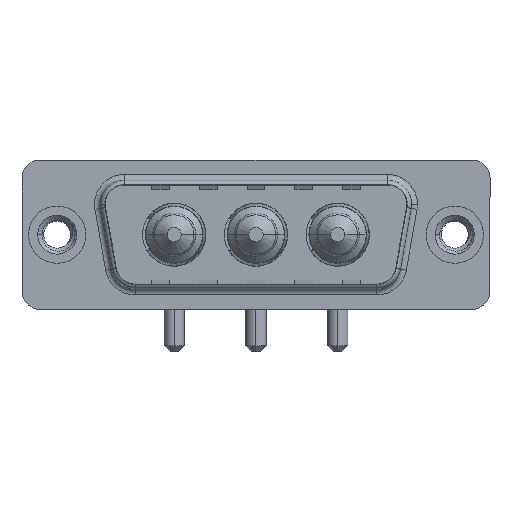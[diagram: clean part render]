
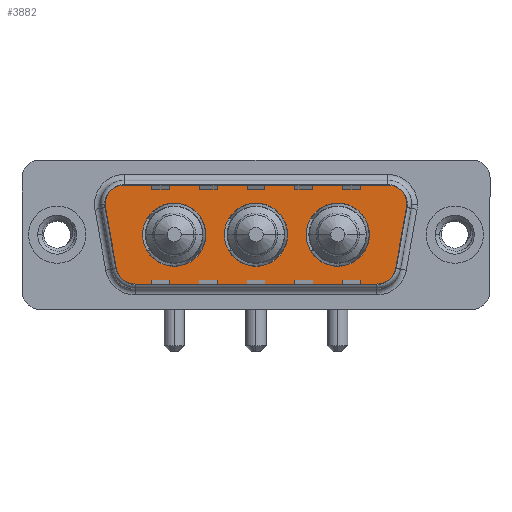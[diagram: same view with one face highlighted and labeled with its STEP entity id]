
A CAD part, top view. The second image highlights one B-rep face of the part: STEP entity #3882.
In plain terms, the highlighted planar face has unit normal (0, 0, 1).
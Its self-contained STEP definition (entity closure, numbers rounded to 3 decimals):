
#53 = VERTEX_POINT ( 'NONE', #10228 ) ;
#57 = CIRCLE ( 'NONE', #4257, 2. ) ;
#200 = LINE ( 'NONE', #8447, #5115 ) ;
#391 = DIRECTION ( 'NONE',  ( 0., 0., 1. ) ) ;
#423 = VERTEX_POINT ( 'NONE', #9043 ) ;
#470 = DIRECTION ( 'NONE',  ( 0., 0., 1. ) ) ;
#472 = ORIENTED_EDGE ( 'NONE', *, *, #7137, .T. ) ;
#653 = DIRECTION ( 'NONE',  ( 1., 0., 0. ) ) ;
#720 = DIRECTION ( 'NONE',  ( 0., 0., 1. ) ) ;
#724 = CARTESIAN_POINT ( 'NONE',  ( 29.889, 2.9, 0. ) ) ;
#821 = DIRECTION ( 'NONE',  ( 0.174, -0.985, 0. ) ) ;
#899 = EDGE_CURVE ( 'NONE', #12222, #423, #8893, .T. ) ;
#1100 = ORIENTED_EDGE ( 'NONE', *, *, #10562, .T. ) ;
#1119 = DIRECTION ( 'NONE',  ( 0., 0., 1. ) ) ;
#1127 = EDGE_CURVE ( 'NONE', #53, #10323, #12072, .T. ) ;
#1172 = VERTEX_POINT ( 'NONE', #9484 ) ;
#1194 = VERTEX_POINT ( 'NONE', #7641 ) ;
#1213 = CARTESIAN_POINT ( 'NONE',  ( 19.3, 0., 0. ) ) ;
#1231 = CARTESIAN_POINT ( 'NONE',  ( 27.889, 2.9, 0. ) ) ;
#1315 = AXIS2_PLACEMENT_3D ( 'NONE', #7459, #3462, #12271 ) ;
#1325 = ORIENTED_EDGE ( 'NONE', *, *, #9516, .T. ) ;
#1352 = DIRECTION ( 'NONE',  ( 0., 0., 1. ) ) ;
#1483 = DIRECTION ( 'NONE',  ( 0., 0., 1. ) ) ;
#1985 = EDGE_LOOP ( 'NONE', ( #4484, #9742, #11621, #472, #1325, #1100, #3845, #10124, #11089 ) ) ;
#2003 = EDGE_CURVE ( 'NONE', #4268, #53, #12152, .T. ) ;
#2082 = EDGE_LOOP ( 'NONE', ( #2613, #12776 ) ) ;
#2243 = CIRCLE ( 'NONE', #12680, 2. ) ;
#2296 = DIRECTION ( 'NONE',  ( 1., 0., 0. ) ) ;
#2495 = EDGE_CURVE ( 'NONE', #10323, #10774, #57, .T. ) ;
#2613 = ORIENTED_EDGE ( 'NONE', *, *, #11477, .F. ) ;
#2951 = CARTESIAN_POINT ( 'NONE',  ( 6.434, -2.9, 0. ) ) ;
#3072 = EDGE_LOOP ( 'NONE', ( #3580, #4823 ) ) ;
#3118 = CARTESIAN_POINT ( 'NONE',  ( 29.859, 2.553, 0. ) ) ;
#3119 = CARTESIAN_POINT ( 'NONE',  ( 27.889, 2.9, 0. ) ) ;
#3271 = VERTEX_POINT ( 'NONE', #10683 ) ;
#3322 = EDGE_CURVE ( 'NONE', #10455, #1172, #9067, .T. ) ;
#3462 = DIRECTION ( 'NONE',  ( 0., 0., 1. ) ) ;
#3522 = VERTEX_POINT ( 'NONE', #5904 ) ;
#3580 = ORIENTED_EDGE ( 'NONE', *, *, #3322, .F. ) ;
#3589 = AXIS2_PLACEMENT_3D ( 'NONE', #9279, #6401, #6276 ) ;
#3667 = CARTESIAN_POINT ( 'NONE',  ( 12.45, 0., 0. ) ) ;
#3845 = ORIENTED_EDGE ( 'NONE', *, *, #899, .T. ) ;
#3882 = ADVANCED_FACE ( 'NONE', ( #8510, #4590, #5574, #10601 ), #12532, .T. ) ;
#4057 = CIRCLE ( 'NONE', #1315, 2.65 ) ;
#4197 = DIRECTION ( 'NONE',  ( -1., 0., 0. ) ) ;
#4220 = DIRECTION ( 'NONE',  ( 0., 0., 1. ) ) ;
#4257 = AXIS2_PLACEMENT_3D ( 'NONE', #3119, #1352, #7123 ) ;
#4268 = VERTEX_POINT ( 'NONE', #12233 ) ;
#4284 = CARTESIAN_POINT ( 'NONE',  ( 26.866, -2.9, 0. ) ) ;
#4433 = VECTOR ( 'NONE', #821, 1000. ) ;
#4484 = ORIENTED_EDGE ( 'NONE', *, *, #2003, .T. ) ;
#4590 = FACE_BOUND ( 'NONE', #2082, .T. ) ;
#4734 = CARTESIAN_POINT ( 'NONE',  ( 23.5, 0., 0. ) ) ;
#4823 = ORIENTED_EDGE ( 'NONE', *, *, #5151, .F. ) ;
#4904 = AXIS2_PLACEMENT_3D ( 'NONE', #4734, #720, #5718 ) ;
#4974 = CARTESIAN_POINT ( 'NONE',  ( 3.441, 2.553, 0. ) ) ;
#5115 = VECTOR ( 'NONE', #6367, 1000. ) ;
#5151 = EDGE_CURVE ( 'NONE', #1172, #10455, #9544, .T. ) ;
#5320 = VERTEX_POINT ( 'NONE', #3667 ) ;
#5481 = AXIS2_PLACEMENT_3D ( 'NONE', #2951, #10925, #9769 ) ;
#5530 = CARTESIAN_POINT ( 'NONE',  ( 7.15, 0., 0. ) ) ;
#5574 = FACE_BOUND ( 'NONE', #6888, .T. ) ;
#5718 = DIRECTION ( 'NONE',  ( 1., 0., 0. ) ) ;
#5741 = VERTEX_POINT ( 'NONE', #7328 ) ;
#5904 = CARTESIAN_POINT ( 'NONE',  ( 27.889, 4.9, 0. ) ) ;
#5947 = AXIS2_PLACEMENT_3D ( 'NONE', #7454, #10639, #11424 ) ;
#6118 = CARTESIAN_POINT ( 'NONE',  ( 16.65, 0., 0. ) ) ;
#6276 = DIRECTION ( 'NONE',  ( 1., 0., 0. ) ) ;
#6367 = DIRECTION ( 'NONE',  ( -1., 0., 0. ) ) ;
#6401 = DIRECTION ( 'NONE',  ( 0., 0., 1. ) ) ;
#6535 = AXIS2_PLACEMENT_3D ( 'NONE', #4284, #1119, #7152 ) ;
#6554 = AXIS2_PLACEMENT_3D ( 'NONE', #6118, #4220, #2296 ) ;
#6616 = LINE ( 'NONE', #9690, #11224 ) ;
#6872 = EDGE_CURVE ( 'NONE', #12348, #4268, #6616, .T. ) ;
#6888 = EDGE_LOOP ( 'NONE', ( #12251, #11708 ) ) ;
#7120 = DIRECTION ( 'NONE',  ( 0.174, 0.985, 0. ) ) ;
#7123 = DIRECTION ( 'NONE',  ( -1., 0., 0. ) ) ;
#7137 = EDGE_CURVE ( 'NONE', #10774, #3522, #2243, .T. ) ;
#7152 = DIRECTION ( 'NONE',  ( 1., 0., 0. ) ) ;
#7236 = AXIS2_PLACEMENT_3D ( 'NONE', #11442, #391, #11312 ) ;
#7328 = CARTESIAN_POINT ( 'NONE',  ( 20.85, 0., 0. ) ) ;
#7389 = CARTESIAN_POINT ( 'NONE',  ( 3.441, 2.553, 0. ) ) ;
#7454 = CARTESIAN_POINT ( 'NONE',  ( 9.8, 0., 0. ) ) ;
#7459 = CARTESIAN_POINT ( 'NONE',  ( 23.5, 0., 0. ) ) ;
#7599 = CARTESIAN_POINT ( 'NONE',  ( 26.866, -2.9, 0. ) ) ;
#7641 = CARTESIAN_POINT ( 'NONE',  ( 26.15, 0., 0. ) ) ;
#8039 = CIRCLE ( 'NONE', #5947, 2.65 ) ;
#8447 = CARTESIAN_POINT ( 'NONE',  ( 5.411, 4.9, 0. ) ) ;
#8510 = FACE_BOUND ( 'NONE', #3072, .T. ) ;
#8579 = DIRECTION ( 'NONE',  ( 1., 0., 0. ) ) ;
#8893 = LINE ( 'NONE', #4974, #4433 ) ;
#9043 = CARTESIAN_POINT ( 'NONE',  ( 4.464, -3.247, 0. ) ) ;
#9067 = CIRCLE ( 'NONE', #6554, 2.65 ) ;
#9068 = VERTEX_POINT ( 'NONE', #5530 ) ;
#9159 = EDGE_CURVE ( 'NONE', #9068, #5320, #12724, .T. ) ;
#9279 = CARTESIAN_POINT ( 'NONE',  ( 5.411, 2.9, 0. ) ) ;
#9484 = CARTESIAN_POINT ( 'NONE',  ( 14., 0., 0. ) ) ;
#9516 = EDGE_CURVE ( 'NONE', #3522, #3271, #200, .T. ) ;
#9544 = CIRCLE ( 'NONE', #7236, 2.65 ) ;
#9690 = CARTESIAN_POINT ( 'NONE',  ( 6.434, -4.9, 0. ) ) ;
#9742 = ORIENTED_EDGE ( 'NONE', *, *, #1127, .T. ) ;
#9769 = DIRECTION ( 'NONE',  ( -1., 0., 0. ) ) ;
#10124 = ORIENTED_EDGE ( 'NONE', *, *, #10663, .T. ) ;
#10228 = CARTESIAN_POINT ( 'NONE',  ( 28.836, -3.247, 0. ) ) ;
#10323 = VERTEX_POINT ( 'NONE', #11625 ) ;
#10454 = AXIS2_PLACEMENT_3D ( 'NONE', #11399, #470, #653 ) ;
#10455 = VERTEX_POINT ( 'NONE', #1213 ) ;
#10481 = VECTOR ( 'NONE', #7120, 1000. ) ;
#10562 = EDGE_CURVE ( 'NONE', #3271, #12222, #12341, .T. ) ;
#10601 = FACE_OUTER_BOUND ( 'NONE', #1985, .T. ) ;
#10639 = DIRECTION ( 'NONE',  ( 0., 0., 1. ) ) ;
#10663 = EDGE_CURVE ( 'NONE', #423, #12348, #11097, .T. ) ;
#10683 = CARTESIAN_POINT ( 'NONE',  ( 5.411, 4.9, 0. ) ) ;
#10774 = VERTEX_POINT ( 'NONE', #724 ) ;
#10925 = DIRECTION ( 'NONE',  ( 0., 0., 1. ) ) ;
#11089 = ORIENTED_EDGE ( 'NONE', *, *, #6872, .T. ) ;
#11097 = CIRCLE ( 'NONE', #5481, 2. ) ;
#11224 = VECTOR ( 'NONE', #8579, 1000. ) ;
#11312 = DIRECTION ( 'NONE',  ( 1., 0., 0. ) ) ;
#11377 = DIRECTION ( 'NONE',  ( 0., 0., 1. ) ) ;
#11399 = CARTESIAN_POINT ( 'NONE',  ( 9.8, 0., 0. ) ) ;
#11424 = DIRECTION ( 'NONE',  ( 1., 0., 0. ) ) ;
#11442 = CARTESIAN_POINT ( 'NONE',  ( 16.65, 0., 0. ) ) ;
#11477 = EDGE_CURVE ( 'NONE', #1194, #5741, #4057, .T. ) ;
#11574 = DIRECTION ( 'NONE',  ( 1., 0., 0. ) ) ;
#11621 = ORIENTED_EDGE ( 'NONE', *, *, #2495, .T. ) ;
#11625 = CARTESIAN_POINT ( 'NONE',  ( 29.859, 2.553, 0. ) ) ;
#11708 = ORIENTED_EDGE ( 'NONE', *, *, #9159, .F. ) ;
#12072 = LINE ( 'NONE', #3118, #10481 ) ;
#12152 = CIRCLE ( 'NONE', #6535, 2. ) ;
#12222 = VERTEX_POINT ( 'NONE', #7389 ) ;
#12233 = CARTESIAN_POINT ( 'NONE',  ( 26.866, -4.9, 0. ) ) ;
#12251 = ORIENTED_EDGE ( 'NONE', *, *, #12419, .F. ) ;
#12271 = DIRECTION ( 'NONE',  ( 1., 0., 0. ) ) ;
#12341 = CIRCLE ( 'NONE', #3589, 2. ) ;
#12348 = VERTEX_POINT ( 'NONE', #12649 ) ;
#12419 = EDGE_CURVE ( 'NONE', #5320, #9068, #8039, .T. ) ;
#12498 = EDGE_CURVE ( 'NONE', #5741, #1194, #12628, .T. ) ;
#12532 = PLANE ( 'NONE',  #12826 ) ;
#12628 = CIRCLE ( 'NONE', #4904, 2.65 ) ;
#12649 = CARTESIAN_POINT ( 'NONE',  ( 6.434, -4.9, 0. ) ) ;
#12680 = AXIS2_PLACEMENT_3D ( 'NONE', #1231, #1483, #4197 ) ;
#12724 = CIRCLE ( 'NONE', #10454, 2.65 ) ;
#12776 = ORIENTED_EDGE ( 'NONE', *, *, #12498, .F. ) ;
#12826 = AXIS2_PLACEMENT_3D ( 'NONE', #7599, #11377, #11574 ) ;
